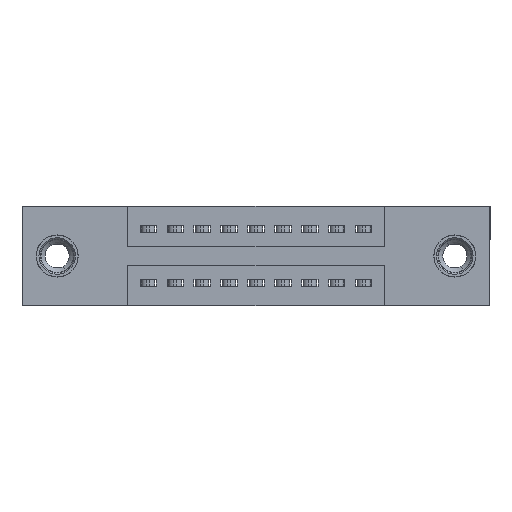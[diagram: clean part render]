
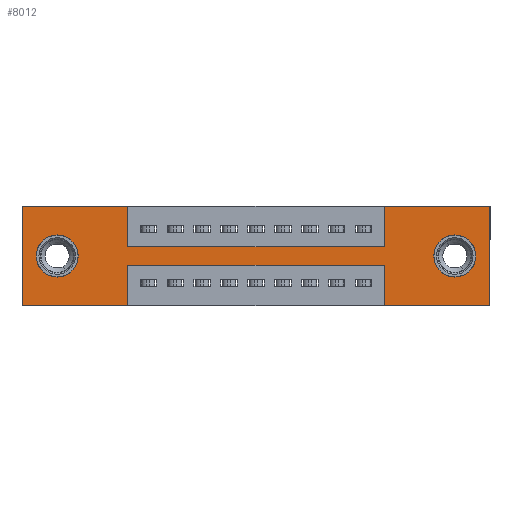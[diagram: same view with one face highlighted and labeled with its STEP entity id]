
A CAD part, front view. The second image highlights one B-rep face of the part: STEP entity #8012.
In plain terms, the highlighted planar face has unit normal (0, -1, 0).
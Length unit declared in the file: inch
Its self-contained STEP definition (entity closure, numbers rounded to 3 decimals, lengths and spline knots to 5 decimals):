
#24 = CARTESIAN_POINT ( 'NONE',  ( 0.3925, 0., 0. ) ) ;
#126 = EDGE_LOOP ( 'NONE', ( #8161, #10676 ) ) ;
#272 = CIRCLE ( 'NONE', #10905, 0.078 ) ;
#279 = VECTOR ( 'NONE', #1568, 39.37008 ) ;
#300 = VECTOR ( 'NONE', #1507, 39.37008 ) ;
#335 = VECTOR ( 'NONE', #9839, 39.37008 ) ;
#370 = LINE ( 'NONE', #3606, #6261 ) ;
#379 = CARTESIAN_POINT ( 'NONE',  ( 0., 0., -0.37 ) ) ;
#419 = LINE ( 'NONE', #9808, #13494 ) ;
#725 = EDGE_CURVE ( 'NONE', #13091, #2685, #2438, .T. ) ;
#843 = CARTESIAN_POINT ( 'NONE',  ( 1.3425, 0., 0. ) ) ;
#1105 = CARTESIAN_POINT ( 'NONE',  ( 0.3925, 0., 0. ) ) ;
#1246 = VECTOR ( 'NONE', #9408, 39.37008 ) ;
#1361 = CARTESIAN_POINT ( 'NONE',  ( 1.735, 0., 0. ) ) ;
#1507 = DIRECTION ( 'NONE',  ( -1., 0., 0. ) ) ;
#1568 = DIRECTION ( 'NONE',  ( -1., 0., 0. ) ) ;
#1649 = VECTOR ( 'NONE', #2681, 39.37008 ) ;
#1709 = FACE_OUTER_BOUND ( 'NONE', #6358, .T. ) ;
#1859 = VECTOR ( 'NONE', #6405, 39.37008 ) ;
#2030 = ORIENTED_EDGE ( 'NONE', *, *, #725, .F. ) ;
#2124 = DIRECTION ( 'NONE',  ( 0., -1., 0. ) ) ;
#2330 = DIRECTION ( 'NONE',  ( 0., 1., 0. ) ) ;
#2438 = LINE ( 'NONE', #8587, #1246 ) ;
#2681 = DIRECTION ( 'NONE',  ( -1., 0., 0. ) ) ;
#2685 = VERTEX_POINT ( 'NONE', #9818 ) ;
#2709 = CARTESIAN_POINT ( 'NONE',  ( 1.605, 0., -0.263 ) ) ;
#2880 = CARTESIAN_POINT ( 'NONE',  ( 0., 0., 0. ) ) ;
#3087 = LINE ( 'NONE', #14805, #4073 ) ;
#3096 = VERTEX_POINT ( 'NONE', #3149 ) ;
#3149 = CARTESIAN_POINT ( 'NONE',  ( 0.3925, 0., -0.37 ) ) ;
#3227 = LINE ( 'NONE', #14098, #12560 ) ;
#3333 = AXIS2_PLACEMENT_3D ( 'NONE', #11300, #12577, #5110 ) ;
#3392 = DIRECTION ( 'NONE',  ( 0., 1., 0. ) ) ;
#3555 = EDGE_CURVE ( 'NONE', #11132, #11521, #370, .T. ) ;
#3606 = CARTESIAN_POINT ( 'NONE',  ( 0., 0., 0. ) ) ;
#3691 = CARTESIAN_POINT ( 'NONE',  ( 1.3425, 0., -0.37 ) ) ;
#3733 = VERTEX_POINT ( 'NONE', #4067 ) ;
#3862 = VERTEX_POINT ( 'NONE', #5836 ) ;
#4067 = CARTESIAN_POINT ( 'NONE',  ( 1.605, 0., -0.107 ) ) ;
#4073 = VECTOR ( 'NONE', #12414, 39.37008 ) ;
#4079 = DIRECTION ( 'NONE',  ( 0., 0., 1. ) ) ;
#4174 = VERTEX_POINT ( 'NONE', #15478 ) ;
#4218 = ORIENTED_EDGE ( 'NONE', *, *, #15559, .F. ) ;
#4451 = CARTESIAN_POINT ( 'NONE',  ( 1.605, 0., -0.185 ) ) ;
#4554 = AXIS2_PLACEMENT_3D ( 'NONE', #4451, #3392, #13346 ) ;
#4643 = VERTEX_POINT ( 'NONE', #5416 ) ;
#4797 = LINE ( 'NONE', #24, #1859 ) ;
#4918 = VERTEX_POINT ( 'NONE', #13624 ) ;
#5110 = DIRECTION ( 'NONE',  ( 0., 0., 1. ) ) ;
#5375 = LINE ( 'NONE', #15183, #1649 ) ;
#5416 = CARTESIAN_POINT ( 'NONE',  ( 0.3925, 0., -0.22 ) ) ;
#5501 = EDGE_CURVE ( 'NONE', #10276, #7339, #3087, .T. ) ;
#5795 = LINE ( 'NONE', #1361, #5981 ) ;
#5836 = CARTESIAN_POINT ( 'NONE',  ( 1.735, 0., -0.37 ) ) ;
#5972 = FACE_BOUND ( 'NONE', #12641, .T. ) ;
#5981 = VECTOR ( 'NONE', #6521, 39.37008 ) ;
#6261 = VECTOR ( 'NONE', #11127, 39.37008 ) ;
#6358 = EDGE_LOOP ( 'NONE', ( #13601, #6810, #2030, #15106, #6921, #13724, #9921, #14347, #14795, #13639, #4218, #12470 ) ) ;
#6391 = LINE ( 'NONE', #7678, #300 ) ;
#6405 = DIRECTION ( 'NONE',  ( 0., 0., -1. ) ) ;
#6435 = EDGE_CURVE ( 'NONE', #9261, #3862, #5795, .T. ) ;
#6521 = DIRECTION ( 'NONE',  ( 0., 0., -1. ) ) ;
#6625 = VERTEX_POINT ( 'NONE', #2709 ) ;
#6782 = EDGE_CURVE ( 'NONE', #3862, #13091, #14569, .T. ) ;
#6810 = ORIENTED_EDGE ( 'NONE', *, *, #16084, .F. ) ;
#6921 = ORIENTED_EDGE ( 'NONE', *, *, #6435, .F. ) ;
#6936 = VECTOR ( 'NONE', #10963, 39.37008 ) ;
#7157 = DIRECTION ( 'NONE',  ( 0., 0., -1. ) ) ;
#7339 = VERTEX_POINT ( 'NONE', #9152 ) ;
#7670 = ORIENTED_EDGE ( 'NONE', *, *, #15990, .T. ) ;
#7678 = CARTESIAN_POINT ( 'NONE',  ( 0., 0., -0.37 ) ) ;
#8012 = ADVANCED_FACE ( 'NONE', ( #13751, #5972, #1709 ), #14460, .T. ) ;
#8161 = ORIENTED_EDGE ( 'NONE', *, *, #9578, .T. ) ;
#8241 = CARTESIAN_POINT ( 'NONE',  ( 0., 0., -0.37 ) ) ;
#8490 = CARTESIAN_POINT ( 'NONE',  ( 0.3925, 0., -0.15 ) ) ;
#8587 = CARTESIAN_POINT ( 'NONE',  ( 1.3425, 0., -0.37 ) ) ;
#9152 = CARTESIAN_POINT ( 'NONE',  ( 1.3425, 0., -0.15 ) ) ;
#9261 = VERTEX_POINT ( 'NONE', #13896 ) ;
#9408 = DIRECTION ( 'NONE',  ( 0., 0., 1. ) ) ;
#9578 = EDGE_CURVE ( 'NONE', #3733, #6625, #272, .T. ) ;
#9591 = EDGE_CURVE ( 'NONE', #7339, #4918, #9862, .T. ) ;
#9791 = CARTESIAN_POINT ( 'NONE',  ( 0.13, 0., -0.185 ) ) ;
#9808 = CARTESIAN_POINT ( 'NONE',  ( 0., 0., 0. ) ) ;
#9818 = CARTESIAN_POINT ( 'NONE',  ( 1.3425, 0., -0.22 ) ) ;
#9839 = DIRECTION ( 'NONE',  ( 0., 0., -1. ) ) ;
#9862 = LINE ( 'NONE', #843, #6936 ) ;
#9921 = ORIENTED_EDGE ( 'NONE', *, *, #9591, .F. ) ;
#9965 = CARTESIAN_POINT ( 'NONE',  ( 0., 0., -0.37 ) ) ;
#10276 = VERTEX_POINT ( 'NONE', #8490 ) ;
#10676 = ORIENTED_EDGE ( 'NONE', *, *, #11876, .T. ) ;
#10799 = EDGE_CURVE ( 'NONE', #4918, #9261, #419, .T. ) ;
#10842 = DIRECTION ( 'NONE',  ( 0., 0., -1. ) ) ;
#10905 = AXIS2_PLACEMENT_3D ( 'NONE', #12187, #14631, #7157 ) ;
#10963 = DIRECTION ( 'NONE',  ( 0., 0., 1. ) ) ;
#11049 = DIRECTION ( 'NONE',  ( 0., 0., 1. ) ) ;
#11127 = DIRECTION ( 'NONE',  ( 1., 0., 0. ) ) ;
#11132 = VERTEX_POINT ( 'NONE', #2880 ) ;
#11300 = CARTESIAN_POINT ( 'NONE',  ( 0.13, 0., -0.185 ) ) ;
#11521 = VERTEX_POINT ( 'NONE', #1105 ) ;
#11876 = EDGE_CURVE ( 'NONE', #6625, #3733, #14465, .T. ) ;
#12187 = CARTESIAN_POINT ( 'NONE',  ( 1.605, 0., -0.185 ) ) ;
#12304 = ORIENTED_EDGE ( 'NONE', *, *, #15264, .T. ) ;
#12356 = CIRCLE ( 'NONE', #3333, 0.078 ) ;
#12414 = DIRECTION ( 'NONE',  ( 1., 0., 0. ) ) ;
#12470 = ORIENTED_EDGE ( 'NONE', *, *, #14836, .F. ) ;
#12560 = VECTOR ( 'NONE', #4079, 39.37008 ) ;
#12577 = DIRECTION ( 'NONE',  ( 0., 1., 0. ) ) ;
#12641 = EDGE_LOOP ( 'NONE', ( #7670, #12304 ) ) ;
#13091 = VERTEX_POINT ( 'NONE', #3691 ) ;
#13346 = DIRECTION ( 'NONE',  ( 0., 0., -1. ) ) ;
#13494 = VECTOR ( 'NONE', #14891, 39.37008 ) ;
#13601 = ORIENTED_EDGE ( 'NONE', *, *, #13912, .F. ) ;
#13624 = CARTESIAN_POINT ( 'NONE',  ( 1.3425, 0., 0. ) ) ;
#13639 = ORIENTED_EDGE ( 'NONE', *, *, #3555, .F. ) ;
#13724 = ORIENTED_EDGE ( 'NONE', *, *, #10799, .F. ) ;
#13725 = CARTESIAN_POINT ( 'NONE',  ( 0.3925, 0., -0.37 ) ) ;
#13748 = CIRCLE ( 'NONE', #13976, 0.078 ) ;
#13751 = FACE_BOUND ( 'NONE', #126, .T. ) ;
#13896 = CARTESIAN_POINT ( 'NONE',  ( 1.735, 0., 0. ) ) ;
#13912 = EDGE_CURVE ( 'NONE', #4643, #3096, #15390, .T. ) ;
#13976 = AXIS2_PLACEMENT_3D ( 'NONE', #9791, #2330, #11049 ) ;
#14098 = CARTESIAN_POINT ( 'NONE',  ( 0., 0., 0. ) ) ;
#14289 = VERTEX_POINT ( 'NONE', #15343 ) ;
#14347 = ORIENTED_EDGE ( 'NONE', *, *, #5501, .F. ) ;
#14460 = PLANE ( 'NONE',  #15495 ) ;
#14465 = CIRCLE ( 'NONE', #4554, 0.078 ) ;
#14569 = LINE ( 'NONE', #9965, #279 ) ;
#14631 = DIRECTION ( 'NONE',  ( 0., 1., 0. ) ) ;
#14795 = ORIENTED_EDGE ( 'NONE', *, *, #16051, .F. ) ;
#14805 = CARTESIAN_POINT ( 'NONE',  ( 0.3925, 0., -0.15 ) ) ;
#14836 = EDGE_CURVE ( 'NONE', #3096, #15512, #6391, .T. ) ;
#14891 = DIRECTION ( 'NONE',  ( 1., 0., 0. ) ) ;
#15106 = ORIENTED_EDGE ( 'NONE', *, *, #6782, .F. ) ;
#15183 = CARTESIAN_POINT ( 'NONE',  ( 0.3925, 0., -0.22 ) ) ;
#15264 = EDGE_CURVE ( 'NONE', #14289, #4174, #13748, .T. ) ;
#15343 = CARTESIAN_POINT ( 'NONE',  ( 0.13, 0., -0.263 ) ) ;
#15390 = LINE ( 'NONE', #13725, #335 ) ;
#15478 = CARTESIAN_POINT ( 'NONE',  ( 0.13, 0., -0.107 ) ) ;
#15495 = AXIS2_PLACEMENT_3D ( 'NONE', #8241, #2124, #10842 ) ;
#15512 = VERTEX_POINT ( 'NONE', #379 ) ;
#15559 = EDGE_CURVE ( 'NONE', #15512, #11132, #3227, .T. ) ;
#15990 = EDGE_CURVE ( 'NONE', #4174, #14289, #12356, .T. ) ;
#16051 = EDGE_CURVE ( 'NONE', #11521, #10276, #4797, .T. ) ;
#16084 = EDGE_CURVE ( 'NONE', #2685, #4643, #5375, .T. ) ;
